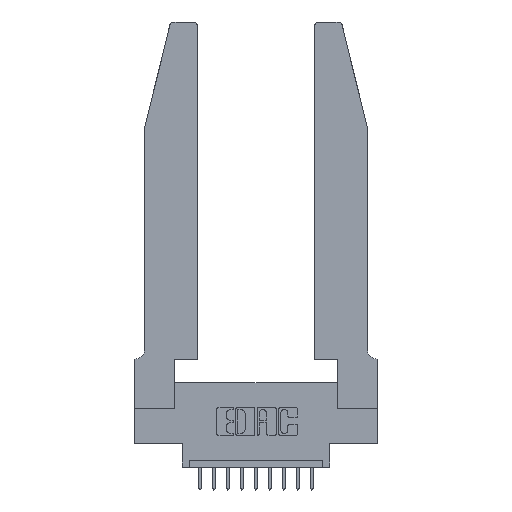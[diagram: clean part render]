
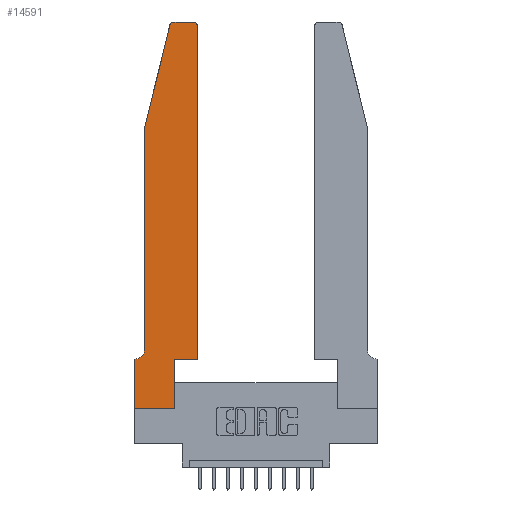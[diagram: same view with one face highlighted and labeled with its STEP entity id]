
A CAD part, top view. The second image highlights one B-rep face of the part: STEP entity #14591.
In plain terms, the highlighted planar face has unit normal (0, 0, 1).
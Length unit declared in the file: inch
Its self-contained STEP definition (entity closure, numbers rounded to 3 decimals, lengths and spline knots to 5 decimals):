
#53 = VERTEX_POINT ( 'NONE', #3609 ) ;
#71 = ORIENTED_EDGE ( 'NONE', *, *, #10339, .T. ) ;
#238 = DIRECTION ( 'NONE',  ( -1., 0., 0. ) ) ;
#538 = AXIS2_PLACEMENT_3D ( 'NONE', #7355, #9686, #2351 ) ;
#576 = DIRECTION ( 'NONE',  ( 0., 0., 1. ) ) ;
#759 = CARTESIAN_POINT ( 'NONE',  ( 0.0755, 2., 0.37 ) ) ;
#1092 = CARTESIAN_POINT ( 'NONE',  ( 0.2605, 2.75, 0.37 ) ) ;
#1762 = DIRECTION ( 'NONE',  ( 0., -1., 0. ) ) ;
#1905 = VECTOR ( 'NONE', #1762, 39.37008 ) ;
#1980 = VERTEX_POINT ( 'NONE', #5255 ) ;
#2075 = LINE ( 'NONE', #6249, #3828 ) ;
#2351 = DIRECTION ( 'NONE',  ( -1., 0., 0. ) ) ;
#2440 = DIRECTION ( 'NONE',  ( 0., 1., 0. ) ) ;
#2530 = LINE ( 'NONE', #759, #7832 ) ;
#2593 = VERTEX_POINT ( 'NONE', #4332 ) ;
#2633 = AXIS2_PLACEMENT_3D ( 'NONE', #9434, #576, #11965 ) ;
#2796 = ORIENTED_EDGE ( 'NONE', *, *, #15697, .T. ) ;
#2868 = EDGE_CURVE ( 'NONE', #4883, #9426, #16167, .T. ) ;
#2891 = VERTEX_POINT ( 'NONE', #9352 ) ;
#3465 = CARTESIAN_POINT ( 'NONE',  ( 0.4505, 2.72, 0.37 ) ) ;
#3609 = CARTESIAN_POINT ( 'NONE',  ( 0.25487, 2.72718, 0.37 ) ) ;
#3828 = VECTOR ( 'NONE', #13687, 39.37008 ) ;
#3855 = CARTESIAN_POINT ( 'NONE',  ( 0.2865, 0.35, 0.37 ) ) ;
#3869 = CARTESIAN_POINT ( 'NONE',  ( 0., 0.35, 0.37 ) ) ;
#3954 = DIRECTION ( 'NONE',  ( -0.239, -0.971, 0. ) ) ;
#4056 = EDGE_CURVE ( 'NONE', #2891, #8447, #14411, .T. ) ;
#4164 = VERTEX_POINT ( 'NONE', #13556 ) ;
#4194 = ORIENTED_EDGE ( 'NONE', *, *, #2868, .T. ) ;
#4332 = CARTESIAN_POINT ( 'NONE',  ( 0.0755, 0.42, 0.37 ) ) ;
#4565 = ORIENTED_EDGE ( 'NONE', *, *, #12724, .T. ) ;
#4722 = ORIENTED_EDGE ( 'NONE', *, *, #4056, .T. ) ;
#4772 = ORIENTED_EDGE ( 'NONE', *, *, #13386, .T. ) ;
#4883 = VERTEX_POINT ( 'NONE', #3869 ) ;
#5023 = DIRECTION ( 'NONE',  ( 1., 0., 0. ) ) ;
#5149 = EDGE_CURVE ( 'NONE', #4164, #9117, #2075, .T. ) ;
#5255 = CARTESIAN_POINT ( 'NONE',  ( 0.0755, 2., 0.37 ) ) ;
#5506 = EDGE_CURVE ( 'NONE', #8846, #4164, #9100, .T. ) ;
#5694 = CARTESIAN_POINT ( 'NONE',  ( 0.4505, 0.35, 0.37 ) ) ;
#5728 = CARTESIAN_POINT ( 'NONE',  ( 0.0055, 0.35, 0.37 ) ) ;
#5798 = VECTOR ( 'NONE', #9928, 39.37008 ) ;
#6084 = AXIS2_PLACEMENT_3D ( 'NONE', #11475, #12454, #5023 ) ;
#6249 = CARTESIAN_POINT ( 'NONE',  ( 0.4505, 0.35, 0.37 ) ) ;
#6754 = ORIENTED_EDGE ( 'NONE', *, *, #5149, .T. ) ;
#7100 = DIRECTION ( 'NONE',  ( 1., 0., 0. ) ) ;
#7160 = CARTESIAN_POINT ( 'NONE',  ( 0.0755, 2., 0.37 ) ) ;
#7185 = CARTESIAN_POINT ( 'NONE',  ( 0., 0., 0.37 ) ) ;
#7355 = CARTESIAN_POINT ( 'NONE',  ( 0.0055, 0.42, 0.37 ) ) ;
#7577 = LINE ( 'NONE', #9725, #15190 ) ;
#7783 = EDGE_CURVE ( 'NONE', #9117, #2891, #12165, .T. ) ;
#7832 = VECTOR ( 'NONE', #3954, 39.37008 ) ;
#8074 = PLANE ( 'NONE',  #2633 ) ;
#8193 = FACE_OUTER_BOUND ( 'NONE', #12461, .T. ) ;
#8238 = ORIENTED_EDGE ( 'NONE', *, *, #13415, .T. ) ;
#8447 = VERTEX_POINT ( 'NONE', #14412 ) ;
#8846 = VERTEX_POINT ( 'NONE', #15267 ) ;
#9100 = LINE ( 'NONE', #5694, #11868 ) ;
#9117 = VERTEX_POINT ( 'NONE', #3465 ) ;
#9204 = LINE ( 'NONE', #7160, #13939 ) ;
#9352 = CARTESIAN_POINT ( 'NONE',  ( 0.4205, 2.75, 0.37 ) ) ;
#9426 = VERTEX_POINT ( 'NONE', #7185 ) ;
#9434 = CARTESIAN_POINT ( 'NONE',  ( 0., 0.35, 0.37 ) ) ;
#9614 = DIRECTION ( 'NONE',  ( 1., 0., 0. ) ) ;
#9686 = DIRECTION ( 'NONE',  ( 0., 0., -1. ) ) ;
#9725 = CARTESIAN_POINT ( 'NONE',  ( 0., 0., 0.37 ) ) ;
#9898 = LINE ( 'NONE', #3855, #16137 ) ;
#9928 = DIRECTION ( 'NONE',  ( -1., 0., 0. ) ) ;
#10089 = VERTEX_POINT ( 'NONE', #14579 ) ;
#10334 = CIRCLE ( 'NONE', #14196, 0.03 ) ;
#10339 = EDGE_CURVE ( 'NONE', #14522, #4883, #13485, .T. ) ;
#10344 = CARTESIAN_POINT ( 'NONE',  ( 0., 0., 0.37 ) ) ;
#10749 = DIRECTION ( 'NONE',  ( 1., 0., 0. ) ) ;
#10758 = CIRCLE ( 'NONE', #538, 0.07 ) ;
#11475 = CARTESIAN_POINT ( 'NONE',  ( 0.4205, 2.72, 0.37 ) ) ;
#11573 = CARTESIAN_POINT ( 'NONE',  ( 0.0755, 0.35, 0.37 ) ) ;
#11868 = VECTOR ( 'NONE', #7100, 39.37008 ) ;
#11891 = ORIENTED_EDGE ( 'NONE', *, *, #14611, .T. ) ;
#11965 = DIRECTION ( 'NONE',  ( 1., 0., 0. ) ) ;
#12063 = CARTESIAN_POINT ( 'NONE',  ( 0.284, 2.72, 0.37 ) ) ;
#12165 = CIRCLE ( 'NONE', #6084, 0.03 ) ;
#12454 = DIRECTION ( 'NONE',  ( 0., 0., 1. ) ) ;
#12461 = EDGE_LOOP ( 'NONE', ( #4722, #11891, #4772, #4565, #8238, #71, #4194, #2796, #12644, #13986, #6754, #15246 ) ) ;
#12644 = ORIENTED_EDGE ( 'NONE', *, *, #15873, .T. ) ;
#12724 = EDGE_CURVE ( 'NONE', #1980, #2593, #9204, .T. ) ;
#13386 = EDGE_CURVE ( 'NONE', #53, #1980, #2530, .T. ) ;
#13415 = EDGE_CURVE ( 'NONE', #2593, #14522, #10758, .T. ) ;
#13485 = LINE ( 'NONE', #11573, #14653 ) ;
#13556 = CARTESIAN_POINT ( 'NONE',  ( 0.4505, 0.35, 0.37 ) ) ;
#13687 = DIRECTION ( 'NONE',  ( 0., 1., 0. ) ) ;
#13939 = VECTOR ( 'NONE', #15768, 39.37008 ) ;
#13986 = ORIENTED_EDGE ( 'NONE', *, *, #5506, .T. ) ;
#14196 = AXIS2_PLACEMENT_3D ( 'NONE', #12063, #15862, #10749 ) ;
#14411 = LINE ( 'NONE', #1092, #5798 ) ;
#14412 = CARTESIAN_POINT ( 'NONE',  ( 0.284, 2.75, 0.37 ) ) ;
#14522 = VERTEX_POINT ( 'NONE', #5728 ) ;
#14579 = CARTESIAN_POINT ( 'NONE',  ( 0.2865, 0., 0.37 ) ) ;
#14591 = ADVANCED_FACE ( 'NONE', ( #8193 ), #8074, .T. ) ;
#14611 = EDGE_CURVE ( 'NONE', #8447, #53, #10334, .T. ) ;
#14653 = VECTOR ( 'NONE', #238, 39.37008 ) ;
#15190 = VECTOR ( 'NONE', #9614, 39.37008 ) ;
#15246 = ORIENTED_EDGE ( 'NONE', *, *, #7783, .T. ) ;
#15267 = CARTESIAN_POINT ( 'NONE',  ( 0.2865, 0.35, 0.37 ) ) ;
#15697 = EDGE_CURVE ( 'NONE', #9426, #10089, #7577, .T. ) ;
#15768 = DIRECTION ( 'NONE',  ( 0., -1., 0. ) ) ;
#15862 = DIRECTION ( 'NONE',  ( 0., 0., 1. ) ) ;
#15873 = EDGE_CURVE ( 'NONE', #10089, #8846, #9898, .T. ) ;
#16137 = VECTOR ( 'NONE', #2440, 39.37008 ) ;
#16167 = LINE ( 'NONE', #10344, #1905 ) ;
